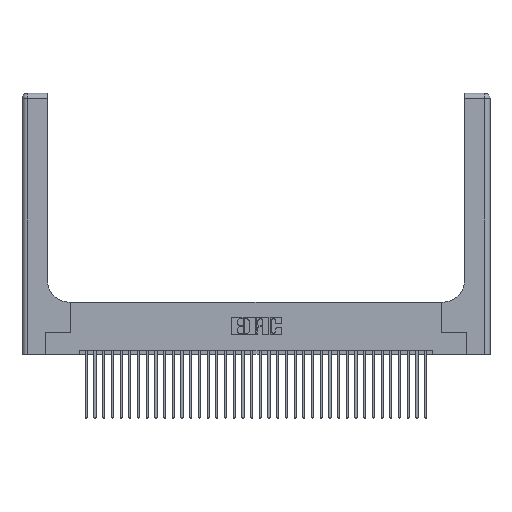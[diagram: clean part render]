
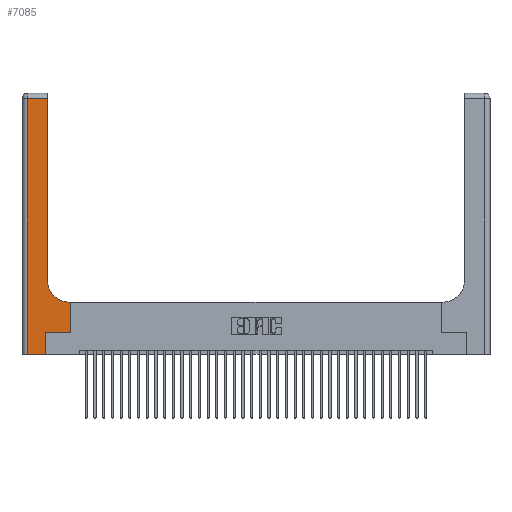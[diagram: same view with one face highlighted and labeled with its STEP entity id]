
A CAD part, top view. The second image highlights one B-rep face of the part: STEP entity #7085.
In plain terms, the highlighted planar face has unit normal (0, 0, 1).
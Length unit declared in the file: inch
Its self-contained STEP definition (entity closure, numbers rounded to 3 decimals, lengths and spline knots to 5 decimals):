
#473 = ORIENTED_EDGE ( 'NONE', *, *, #1234, .T. ) ;
#641 = CARTESIAN_POINT ( 'NONE',  ( 0., 0., 0.37 ) ) ;
#980 = CIRCLE ( 'NONE', #24320, 0.25 ) ;
#1234 = EDGE_CURVE ( 'NONE', #13658, #17238, #980, .T. ) ;
#1640 = ORIENTED_EDGE ( 'NONE', *, *, #10272, .T. ) ;
#2148 = CARTESIAN_POINT ( 'NONE',  ( 0.5585, 0.25, 0.37 ) ) ;
#2334 = EDGE_CURVE ( 'NONE', #21191, #24223, #5866, .T. ) ;
#2858 = DIRECTION ( 'NONE',  ( 0., 1., 0. ) ) ;
#3050 = VECTOR ( 'NONE', #22742, 39.37008 ) ;
#3460 = VECTOR ( 'NONE', #23474, 39.37008 ) ;
#3481 = CARTESIAN_POINT ( 'NONE',  ( 0.2915, 2.94, 0.37 ) ) ;
#3563 = CARTESIAN_POINT ( 'NONE',  ( 0.5585, 0.25, 0.37 ) ) ;
#4139 = VERTEX_POINT ( 'NONE', #22418 ) ;
#4667 = CARTESIAN_POINT ( 'NONE',  ( 0.2915, 0.6, 0.37 ) ) ;
#5555 = CARTESIAN_POINT ( 'NONE',  ( 0.5415, 0.85, 0.37 ) ) ;
#5866 = LINE ( 'NONE', #31179, #11649 ) ;
#7029 = DIRECTION ( 'NONE',  ( -1., 0., 0. ) ) ;
#7062 = EDGE_CURVE ( 'NONE', #8241, #4139, #30765, .T. ) ;
#7080 = ORIENTED_EDGE ( 'NONE', *, *, #7062, .T. ) ;
#7085 = ADVANCED_FACE ( 'NONE', ( #8090 ), #32746, .F. ) ;
#8090 = FACE_OUTER_BOUND ( 'NONE', #19244, .T. ) ;
#8241 = VERTEX_POINT ( 'NONE', #3481 ) ;
#8305 = VECTOR ( 'NONE', #12300, 39.37008 ) ;
#8390 = DIRECTION ( 'NONE',  ( 1., 0., 0. ) ) ;
#8598 = ORIENTED_EDGE ( 'NONE', *, *, #2334, .T. ) ;
#9524 = VERTEX_POINT ( 'NONE', #21164 ) ;
#9648 = LINE ( 'NONE', #30263, #32316 ) ;
#9658 = CARTESIAN_POINT ( 'NONE',  ( 0.5415, 0.6, 0.37 ) ) ;
#9995 = EDGE_CURVE ( 'NONE', #18242, #21191, #18602, .T. ) ;
#10272 = EDGE_CURVE ( 'NONE', #17238, #8241, #9648, .T. ) ;
#11649 = VECTOR ( 'NONE', #2858, 39.37008 ) ;
#11950 = LINE ( 'NONE', #2148, #27079 ) ;
#12300 = DIRECTION ( 'NONE',  ( 1., 0., 0. ) ) ;
#12566 = EDGE_CURVE ( 'NONE', #22321, #9524, #11950, .T. ) ;
#12832 = CARTESIAN_POINT ( 'NONE',  ( 0.269, 0., 0.37 ) ) ;
#13243 = DIRECTION ( 'NONE',  ( 0., 1., 0. ) ) ;
#13606 = EDGE_CURVE ( 'NONE', #24223, #22321, #31856, .T. ) ;
#13658 = VERTEX_POINT ( 'NONE', #9658 ) ;
#14851 = ORIENTED_EDGE ( 'NONE', *, *, #12566, .T. ) ;
#15650 = VECTOR ( 'NONE', #7029, 39.37008 ) ;
#16267 = EDGE_CURVE ( 'NONE', #9524, #13658, #35183, .T. ) ;
#16518 = ORIENTED_EDGE ( 'NONE', *, *, #35702, .T. ) ;
#17238 = VERTEX_POINT ( 'NONE', #29070 ) ;
#18003 = CARTESIAN_POINT ( 'NONE',  ( 0.269, 0.25, 0.37 ) ) ;
#18175 = LINE ( 'NONE', #19878, #3050 ) ;
#18242 = VERTEX_POINT ( 'NONE', #18547 ) ;
#18547 = CARTESIAN_POINT ( 'NONE',  ( 0.06, 0., 0.37 ) ) ;
#18602 = LINE ( 'NONE', #641, #3460 ) ;
#19244 = EDGE_LOOP ( 'NONE', ( #1640, #7080, #16518, #31551, #8598, #28749, #14851, #33718, #473 ) ) ;
#19878 = CARTESIAN_POINT ( 'NONE',  ( 0.06, 3., 0.37 ) ) ;
#21164 = CARTESIAN_POINT ( 'NONE',  ( 0.5585, 0.6, 0.37 ) ) ;
#21191 = VERTEX_POINT ( 'NONE', #12832 ) ;
#21357 = DIRECTION ( 'NONE',  ( 0., 0., -1. ) ) ;
#22321 = VERTEX_POINT ( 'NONE', #3563 ) ;
#22418 = CARTESIAN_POINT ( 'NONE',  ( 0.06, 2.94, 0.37 ) ) ;
#22742 = DIRECTION ( 'NONE',  ( 0., -1., 0. ) ) ;
#23474 = DIRECTION ( 'NONE',  ( 1., 0., 0. ) ) ;
#24223 = VERTEX_POINT ( 'NONE', #25162 ) ;
#24320 = AXIS2_PLACEMENT_3D ( 'NONE', #5555, #25471, #8390 ) ;
#24590 = DIRECTION ( 'NONE',  ( -1., 0., 0. ) ) ;
#25162 = CARTESIAN_POINT ( 'NONE',  ( 0.269, 0.25, 0.37 ) ) ;
#25471 = DIRECTION ( 'NONE',  ( 0., 0., -1. ) ) ;
#26811 = VECTOR ( 'NONE', #24590, 39.37008 ) ;
#27079 = VECTOR ( 'NONE', #36190, 39.37008 ) ;
#28749 = ORIENTED_EDGE ( 'NONE', *, *, #13606, .T. ) ;
#29070 = CARTESIAN_POINT ( 'NONE',  ( 0.2915, 0.85, 0.37 ) ) ;
#29763 = CARTESIAN_POINT ( 'NONE',  ( 0., 2.94, 0.37 ) ) ;
#29887 = CARTESIAN_POINT ( 'NONE',  ( 0., 3., 0.37 ) ) ;
#30263 = CARTESIAN_POINT ( 'NONE',  ( 0.2915, 3., 0.37 ) ) ;
#30765 = LINE ( 'NONE', #29763, #15650 ) ;
#31179 = CARTESIAN_POINT ( 'NONE',  ( 0.269, 0., 0.37 ) ) ;
#31551 = ORIENTED_EDGE ( 'NONE', *, *, #9995, .T. ) ;
#31856 = LINE ( 'NONE', #18003, #8305 ) ;
#32316 = VECTOR ( 'NONE', #13243, 39.37008 ) ;
#32746 = PLANE ( 'NONE',  #33885 ) ;
#33718 = ORIENTED_EDGE ( 'NONE', *, *, #16267, .T. ) ;
#33885 = AXIS2_PLACEMENT_3D ( 'NONE', #29887, #21357, #35561 ) ;
#35183 = LINE ( 'NONE', #4667, #26811 ) ;
#35561 = DIRECTION ( 'NONE',  ( -1., 0., 0. ) ) ;
#35702 = EDGE_CURVE ( 'NONE', #4139, #18242, #18175, .T. ) ;
#36190 = DIRECTION ( 'NONE',  ( 0., 1., 0. ) ) ;
